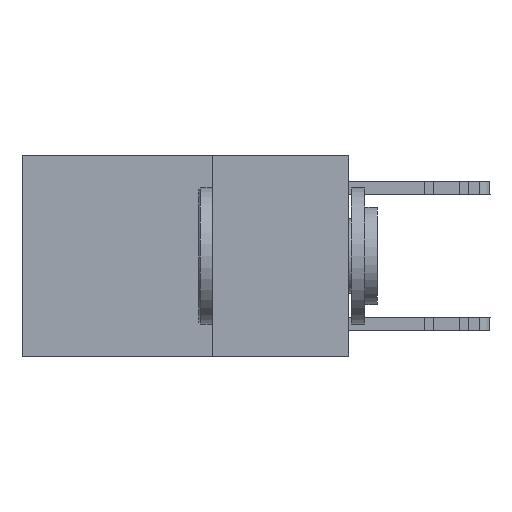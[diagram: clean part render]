
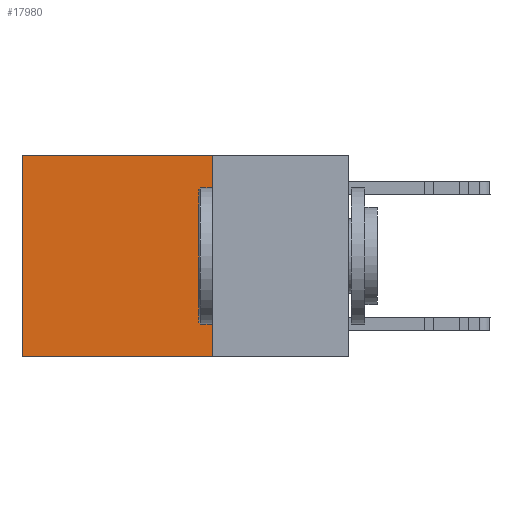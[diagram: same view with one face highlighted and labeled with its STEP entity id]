
A CAD part, left-side view. The second image highlights one B-rep face of the part: STEP entity #17980.
In plain terms, the highlighted planar face has unit normal (-1, 0, 0).
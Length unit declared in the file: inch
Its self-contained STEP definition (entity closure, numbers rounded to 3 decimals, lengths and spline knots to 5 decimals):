
#2928 = VECTOR ( 'NONE', #14801, 39.37008 ) ;
#2974 = VERTEX_POINT ( 'NONE', #8657 ) ;
#3005 = ORIENTED_EDGE ( 'NONE', *, *, #31216, .T. ) ;
#3127 = AXIS2_PLACEMENT_3D ( 'NONE', #29264, #29220, #29200 ) ;
#3313 = LINE ( 'NONE', #15660, #2928 ) ;
#8657 = CARTESIAN_POINT ( 'NONE',  ( 0.2625, 0.25, -0.37 ) ) ;
#9982 = CARTESIAN_POINT ( 'NONE',  ( 0.2625, 0.6, 0. ) ) ;
#10040 = VERTEX_POINT ( 'NONE', #14827 ) ;
#10379 = VECTOR ( 'NONE', #27231, 39.37008 ) ;
#10417 = LINE ( 'NONE', #26401, #10379 ) ;
#11576 = EDGE_CURVE ( 'NONE', #20558, #10040, #10417, .T. ) ;
#11991 = EDGE_CURVE ( 'NONE', #20558, #2974, #3313, .T. ) ;
#12467 = DIRECTION ( 'NONE',  ( 0., 0., -1. ) ) ;
#14801 = DIRECTION ( 'NONE',  ( 0., 0., -1. ) ) ;
#14827 = CARTESIAN_POINT ( 'NONE',  ( 0.2625, 0.6, 0. ) ) ;
#14964 = VECTOR ( 'NONE', #20953, 39.37008 ) ;
#15314 = LINE ( 'NONE', #20764, #14964 ) ;
#15660 = CARTESIAN_POINT ( 'NONE',  ( 0.2625, 0.25, 0. ) ) ;
#16516 = CARTESIAN_POINT ( 'NONE',  ( 0.2625, 0.6, -0.37 ) ) ;
#17737 = ORIENTED_EDGE ( 'NONE', *, *, #11576, .T. ) ;
#17980 = ADVANCED_FACE ( 'NONE', ( #26578 ), #29401, .F. ) ;
#18854 = VERTEX_POINT ( 'NONE', #16516 ) ;
#20558 = VERTEX_POINT ( 'NONE', #30152 ) ;
#20764 = CARTESIAN_POINT ( 'NONE',  ( 0.2625, 0.25, -0.37 ) ) ;
#20953 = DIRECTION ( 'NONE',  ( 0., 1., 0. ) ) ;
#21632 = EDGE_CURVE ( 'NONE', #2974, #18854, #15314, .T. ) ;
#24487 = ORIENTED_EDGE ( 'NONE', *, *, #21632, .F. ) ;
#26401 = CARTESIAN_POINT ( 'NONE',  ( 0.2625, 0.25, 0. ) ) ;
#26578 = FACE_OUTER_BOUND ( 'NONE', #28876, .T. ) ;
#27231 = DIRECTION ( 'NONE',  ( 0., 1., 0. ) ) ;
#28536 = ORIENTED_EDGE ( 'NONE', *, *, #11991, .F. ) ;
#28812 = VECTOR ( 'NONE', #12467, 39.37008 ) ;
#28876 = EDGE_LOOP ( 'NONE', ( #3005, #24487, #28536, #17737 ) ) ;
#29200 = DIRECTION ( 'NONE',  ( 0., 0., -1. ) ) ;
#29220 = DIRECTION ( 'NONE',  ( 1., 0., 0. ) ) ;
#29264 = CARTESIAN_POINT ( 'NONE',  ( 0.2625, 0.25, 0. ) ) ;
#29401 = PLANE ( 'NONE',  #3127 ) ;
#29543 = LINE ( 'NONE', #9982, #28812 ) ;
#30152 = CARTESIAN_POINT ( 'NONE',  ( 0.2625, 0.25, 0. ) ) ;
#31216 = EDGE_CURVE ( 'NONE', #10040, #18854, #29543, .T. ) ;
